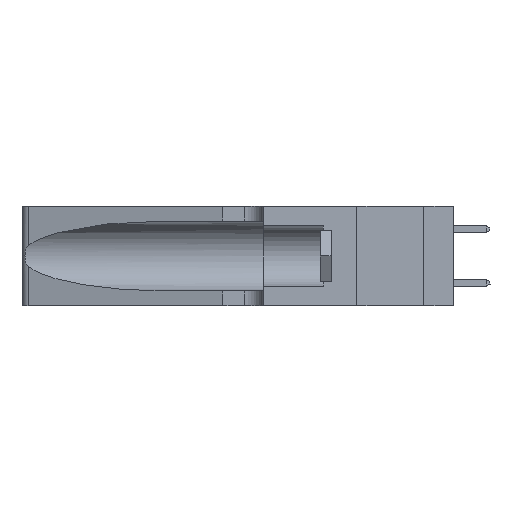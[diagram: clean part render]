
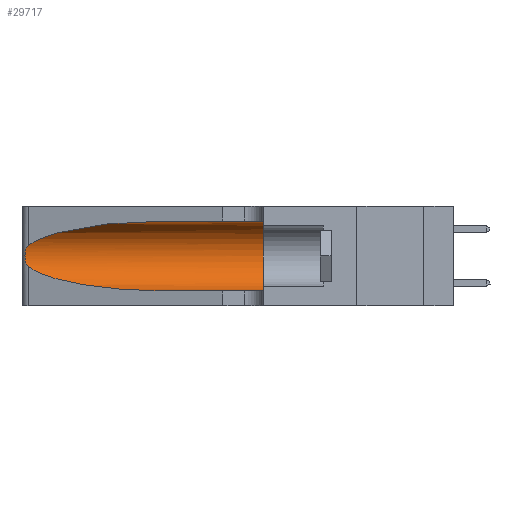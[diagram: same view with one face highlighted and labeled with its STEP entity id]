
A CAD part, left-side view. The second image highlights one B-rep face of the part: STEP entity #29717.
In plain terms, the highlighted cylindrical face has radius 3.308 mm (diameter 6.617 mm), a partial arc.
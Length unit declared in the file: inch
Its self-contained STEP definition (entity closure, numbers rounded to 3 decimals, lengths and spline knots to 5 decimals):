
#702 = CARTESIAN_POINT ( 'NONE',  ( 0.2373, 1.15595, 0.28018 ) ) ;
#1788 = CARTESIAN_POINT ( 'NONE',  ( 0.2373, 1.15595, 0.08982 ) ) ;
#2701 = AXIS2_PLACEMENT_3D ( 'NONE', #39829, #29216, #18726 ) ;
#2925 = CARTESIAN_POINT ( 'NONE',  ( 0.25856, 1.23593, 0.16098 ) ) ;
#4684 =( BOUNDED_CURVE ( )  B_SPLINE_CURVE ( 3, ( #43011, #21894, #702, #25438 ),
 .UNSPECIFIED., .F., .F. ) 
 B_SPLINE_CURVE_WITH_KNOTS ( ( 4, 4 ),
 ( 1.5708, 2.84003 ),
 .UNSPECIFIED. ) 
 CURVE ( )  GEOMETRIC_REPRESENTATION_ITEM ( )  RATIONAL_B_SPLINE_CURVE ( ( 1., 0.87, 0.87, 1. ) ) 
 REPRESENTATION_ITEM ( '' )  );
#6537 = CARTESIAN_POINT ( 'NONE',  ( 0.25639, 1.23186, 0.15144 ) ) ;
#7062 = ORIENTED_EDGE ( 'NONE', *, *, #42230, .T. ) ;
#10080 = CARTESIAN_POINT ( 'NONE',  ( 0.25487, 1.22718, 0.14631 ) ) ;
#10902 = LINE ( 'NONE', #36094, #28545 ) ;
#11069 = ORIENTED_EDGE ( 'NONE', *, *, #40906, .F. ) ;
#12223 = VERTEX_POINT ( 'NONE', #20611 ) ;
#12640 = ORIENTED_EDGE ( 'NONE', *, *, #28486, .T. ) ;
#13482 = CARTESIAN_POINT ( 'NONE',  ( 0.25639, 1.23184, 0.21858 ) ) ;
#13738 = EDGE_CURVE ( 'NONE', #12223, #38095, #32725, .T. ) ;
#14589 = VERTEX_POINT ( 'NONE', #42803 ) ;
#14991 = FACE_OUTER_BOUND ( 'NONE', #19767, .T. ) ;
#17029 = CARTESIAN_POINT ( 'NONE',  ( 0.25854, 1.2359, 0.20912 ) ) ;
#18475 = CARTESIAN_POINT ( 'NONE',  ( 0.1305, 1.61858, 0.31525 ) ) ;
#18635 = CARTESIAN_POINT ( 'NONE',  ( 0.1305, 0.35, 0.185 ) ) ;
#18726 = DIRECTION ( 'NONE',  ( 0., 0., -1. ) ) ;
#18828 = CIRCLE ( 'NONE', #21402, 0.13025 ) ;
#19434 = CARTESIAN_POINT ( 'NONE',  ( 0.1305, 0.72297, 0.31525 ) ) ;
#19587 = CARTESIAN_POINT ( 'NONE',  ( 0.1305, 0.72297, 0.05475 ) ) ;
#19767 = EDGE_LOOP ( 'NONE', ( #7062, #35758, #12640, #31855, #27035, #11069 ) ) ;
#19832 = CARTESIAN_POINT ( 'NONE',  ( 0.1305, 0.35, 0.05475 ) ) ;
#20559 = CARTESIAN_POINT ( 'NONE',  ( 0.26075, 1.23896, 0.19203 ) ) ;
#20611 = CARTESIAN_POINT ( 'NONE',  ( 0.25487, 1.22718, 0.22369 ) ) ;
#21135 = EDGE_CURVE ( 'NONE', #40359, #25029, #10902, .T. ) ;
#21402 = AXIS2_PLACEMENT_3D ( 'NONE', #18635, #43262, #22140 ) ;
#21894 = CARTESIAN_POINT ( 'NONE',  ( 0.18966, 0.96281, 0.31525 ) ) ;
#22140 = DIRECTION ( 'NONE',  ( 0., 0., 1. ) ) ;
#23926 = CARTESIAN_POINT ( 'NONE',  ( 0.25555, 1.22994, 0.2215 ) ) ;
#24095 = CARTESIAN_POINT ( 'NONE',  ( 0.26017, 1.23833, 0.17102 ) ) ;
#25029 = VERTEX_POINT ( 'NONE', #19832 ) ;
#25438 = CARTESIAN_POINT ( 'NONE',  ( 0.25487, 1.22718, 0.22369 ) ) ;
#27035 = ORIENTED_EDGE ( 'NONE', *, *, #45495, .F. ) ;
#27651 = CARTESIAN_POINT ( 'NONE',  ( 0.25789, 1.23486, 0.15765 ) ) ;
#28486 = EDGE_CURVE ( 'NONE', #38095, #40359, #37509, .T. ) ;
#28545 = VECTOR ( 'NONE', #32584, 39.37008 ) ;
#29216 = DIRECTION ( 'NONE',  ( 0., -1., 0. ) ) ;
#29717 = ADVANCED_FACE ( 'NONE', ( #14991 ), #41981, .F. ) ;
#29791 = CARTESIAN_POINT ( 'NONE',  ( 0.1305, 0.72297, 0.05475 ) ) ;
#30089 = CARTESIAN_POINT ( 'NONE',  ( 0.25487, 1.22718, 0.14631 ) ) ;
#31226 = CARTESIAN_POINT ( 'NONE',  ( 0.25555, 1.22993, 0.14849 ) ) ;
#31855 = ORIENTED_EDGE ( 'NONE', *, *, #21135, .T. ) ;
#32584 = DIRECTION ( 'NONE',  ( 0., -1., 0. ) ) ;
#32725 = B_SPLINE_CURVE_WITH_KNOTS ( 'NONE', 3,
 ( #37975, #23926, #13482, #38116, #17029, #41644, #20559, #45173, #24095, #2925, #27651, #6537, #31226, #10080 ),
 .UNSPECIFIED., .F., .F.,
 ( 4, 2, 2, 2, 2, 2, 4 ),
 ( 0., 0.00027, 0.00053, 0.00107, 0.0016, 0.00187, 0.00214 ),
 .UNSPECIFIED. ) ;
#33567 = VECTOR ( 'NONE', #36041, 39.37008 ) ;
#34093 = VERTEX_POINT ( 'NONE', #19434 ) ;
#34680 = LINE ( 'NONE', #18475, #33567 ) ;
#35758 = ORIENTED_EDGE ( 'NONE', *, *, #13738, .T. ) ;
#36041 = DIRECTION ( 'NONE',  ( 0., -1., 0. ) ) ;
#36094 = CARTESIAN_POINT ( 'NONE',  ( 0.1305, 1.61858, 0.05475 ) ) ;
#36161 = CARTESIAN_POINT ( 'NONE',  ( 0.25487, 1.22718, 0.14631 ) ) ;
#37509 =( BOUNDED_CURVE ( )  B_SPLINE_CURVE ( 3, ( #30089, #1788, #40701, #19587 ),
 .UNSPECIFIED., .F., .F. ) 
 B_SPLINE_CURVE_WITH_KNOTS ( ( 4, 4 ),
 ( 3.44316, 4.71239 ),
 .UNSPECIFIED. ) 
 CURVE ( )  GEOMETRIC_REPRESENTATION_ITEM ( )  RATIONAL_B_SPLINE_CURVE ( ( 1., 0.87, 0.87, 1. ) ) 
 REPRESENTATION_ITEM ( '' )  );
#37975 = CARTESIAN_POINT ( 'NONE',  ( 0.25487, 1.22718, 0.22369 ) ) ;
#38095 = VERTEX_POINT ( 'NONE', #36161 ) ;
#38116 = CARTESIAN_POINT ( 'NONE',  ( 0.25787, 1.23484, 0.2124 ) ) ;
#39829 = CARTESIAN_POINT ( 'NONE',  ( 0.1305, 1.61858, 0.185 ) ) ;
#40359 = VERTEX_POINT ( 'NONE', #29791 ) ;
#40701 = CARTESIAN_POINT ( 'NONE',  ( 0.18966, 0.96281, 0.05475 ) ) ;
#40906 = EDGE_CURVE ( 'NONE', #34093, #14589, #34680, .T. ) ;
#41644 = CARTESIAN_POINT ( 'NONE',  ( 0.26018, 1.23835, 0.19895 ) ) ;
#41981 = CYLINDRICAL_SURFACE ( 'NONE', #2701, 0.13025 ) ;
#42230 = EDGE_CURVE ( 'NONE', #34093, #12223, #4684, .T. ) ;
#42803 = CARTESIAN_POINT ( 'NONE',  ( 0.1305, 0.35, 0.31525 ) ) ;
#43011 = CARTESIAN_POINT ( 'NONE',  ( 0.1305, 0.72297, 0.31525 ) ) ;
#43262 = DIRECTION ( 'NONE',  ( 0., 1., 0. ) ) ;
#45173 = CARTESIAN_POINT ( 'NONE',  ( 0.26075, 1.23896, 0.178 ) ) ;
#45495 = EDGE_CURVE ( 'NONE', #14589, #25029, #18828, .T. ) ;
